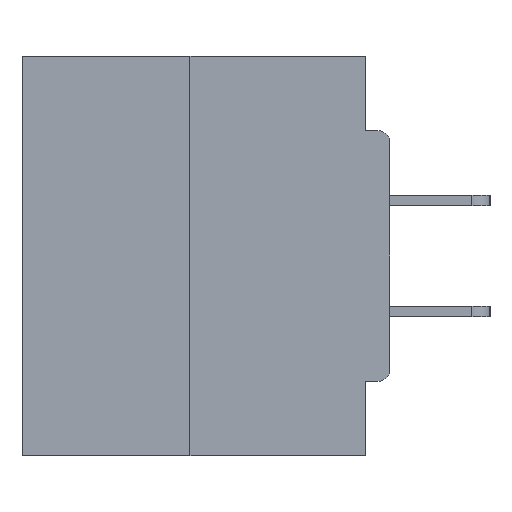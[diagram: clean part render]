
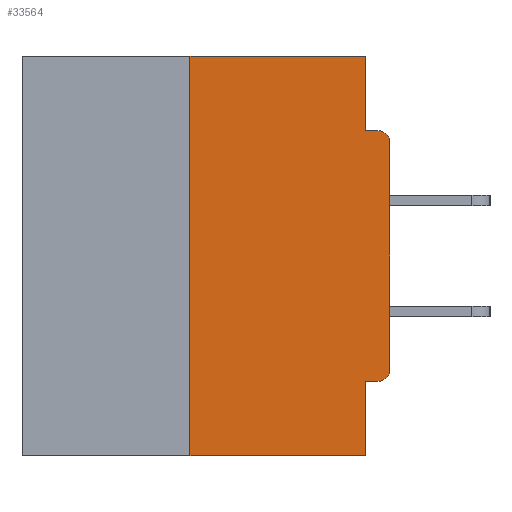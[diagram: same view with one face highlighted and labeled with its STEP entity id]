
A CAD part, left-side view. The second image highlights one B-rep face of the part: STEP entity #33564.
In plain terms, the highlighted planar face has unit normal (-1, 0, 0).
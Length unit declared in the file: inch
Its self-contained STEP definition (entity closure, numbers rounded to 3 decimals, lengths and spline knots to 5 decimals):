
#70 = CIRCLE ( 'NONE', #27551, 0.015 ) ;
#1037 = VERTEX_POINT ( 'NONE', #1949 ) ;
#1400 = LINE ( 'NONE', #12373, #30308 ) ;
#1411 = DIRECTION ( 'NONE',  ( 0., 0., -1. ) ) ;
#1765 = CARTESIAN_POINT ( 'NONE',  ( 0., 0.25, 0. ) ) ;
#1949 = CARTESIAN_POINT ( 'NONE',  ( 0., 0.031, -0.5 ) ) ;
#1954 = CARTESIAN_POINT ( 'NONE',  ( 0., 0.46, 0. ) ) ;
#2030 = EDGE_CURVE ( 'NONE', #9656, #1037, #1400, .T. ) ;
#2289 = ORIENTED_EDGE ( 'NONE', *, *, #35875, .F. ) ;
#2880 = CARTESIAN_POINT ( 'NONE',  ( 0., 0.25, -0.5 ) ) ;
#2998 = VERTEX_POINT ( 'NONE', #32432 ) ;
#3151 = LINE ( 'NONE', #27882, #17383 ) ;
#3451 = CARTESIAN_POINT ( 'NONE',  ( 0., 0.46, 0. ) ) ;
#4517 = DIRECTION ( 'NONE',  ( 1., 0., 0. ) ) ;
#4661 = CARTESIAN_POINT ( 'NONE',  ( 0., 0., -0.4065 ) ) ;
#5572 = ORIENTED_EDGE ( 'NONE', *, *, #20183, .F. ) ;
#7236 = ORIENTED_EDGE ( 'NONE', *, *, #28558, .T. ) ;
#7352 = AXIS2_PLACEMENT_3D ( 'NONE', #29570, #26104, #34522 ) ;
#9108 = DIRECTION ( 'NONE',  ( 0., 0., 1. ) ) ;
#9646 = PLANE ( 'NONE',  #12775 ) ;
#9656 = VERTEX_POINT ( 'NONE', #2880 ) ;
#10022 = VECTOR ( 'NONE', #9108, 39.37008 ) ;
#10520 = LINE ( 'NONE', #4661, #33138 ) ;
#10709 = EDGE_CURVE ( 'NONE', #30648, #2998, #70, .T. ) ;
#10885 = EDGE_CURVE ( 'NONE', #9656, #11603, #18848, .T. ) ;
#11100 = CARTESIAN_POINT ( 'NONE',  ( 0., 0.031, 0. ) ) ;
#11118 = CARTESIAN_POINT ( 'NONE',  ( 0., 0., -0.3915 ) ) ;
#11220 = EDGE_LOOP ( 'NONE', ( #2289, #21263, #24983, #5572, #11323, #7236, #27194, #15880, #24180, #26941 ) ) ;
#11323 = ORIENTED_EDGE ( 'NONE', *, *, #15122, .F. ) ;
#11603 = VERTEX_POINT ( 'NONE', #1765 ) ;
#12114 = CARTESIAN_POINT ( 'NONE',  ( 0., 0.031, -0.4065 ) ) ;
#12373 = CARTESIAN_POINT ( 'NONE',  ( 0., 0.46, -0.5 ) ) ;
#12559 = DIRECTION ( 'NONE',  ( 0., -1., 0. ) ) ;
#12775 = AXIS2_PLACEMENT_3D ( 'NONE', #1954, #4517, #1411 ) ;
#12781 = LINE ( 'NONE', #32939, #34149 ) ;
#14310 = CARTESIAN_POINT ( 'NONE',  ( 0., 0., -0.1085 ) ) ;
#15122 = EDGE_CURVE ( 'NONE', #18452, #19580, #10520, .T. ) ;
#15360 = CARTESIAN_POINT ( 'NONE',  ( 0., 0.015, -0.1085 ) ) ;
#15540 = CIRCLE ( 'NONE', #7352, 0.015 ) ;
#15880 = ORIENTED_EDGE ( 'NONE', *, *, #10709, .T. ) ;
#16033 = CARTESIAN_POINT ( 'NONE',  ( 0., 0.031, -0.0935 ) ) ;
#16152 = EDGE_CURVE ( 'NONE', #31813, #2998, #3151, .T. ) ;
#16269 = EDGE_CURVE ( 'NONE', #17108, #30648, #31341, .T. ) ;
#16673 = VECTOR ( 'NONE', #30691, 39.37008 ) ;
#17108 = VERTEX_POINT ( 'NONE', #11118 ) ;
#17383 = VECTOR ( 'NONE', #30617, 39.37008 ) ;
#17962 = DIRECTION ( 'NONE',  ( 0., 0., 1. ) ) ;
#18189 = CARTESIAN_POINT ( 'NONE',  ( 0., 0.031, 0. ) ) ;
#18452 = VERTEX_POINT ( 'NONE', #28860 ) ;
#18848 = LINE ( 'NONE', #30004, #10022 ) ;
#19001 = LINE ( 'NONE', #11100, #16673 ) ;
#19060 = VERTEX_POINT ( 'NONE', #18189 ) ;
#19580 = VERTEX_POINT ( 'NONE', #12114 ) ;
#20183 = EDGE_CURVE ( 'NONE', #19580, #1037, #12781, .T. ) ;
#21263 = ORIENTED_EDGE ( 'NONE', *, *, #10885, .F. ) ;
#21328 = DIRECTION ( 'NONE',  ( 0., 1., 0. ) ) ;
#23045 = LINE ( 'NONE', #3451, #28576 ) ;
#24147 = DIRECTION ( 'NONE',  ( 0., 0., -1. ) ) ;
#24180 = ORIENTED_EDGE ( 'NONE', *, *, #16152, .F. ) ;
#24983 = ORIENTED_EDGE ( 'NONE', *, *, #2030, .T. ) ;
#26104 = DIRECTION ( 'NONE',  ( -1., 0., 0. ) ) ;
#26484 = FACE_OUTER_BOUND ( 'NONE', #11220, .T. ) ;
#26570 = CARTESIAN_POINT ( 'NONE',  ( 0., 0., 0. ) ) ;
#26941 = ORIENTED_EDGE ( 'NONE', *, *, #28267, .F. ) ;
#27194 = ORIENTED_EDGE ( 'NONE', *, *, #16269, .T. ) ;
#27551 = AXIS2_PLACEMENT_3D ( 'NONE', #15360, #34952, #35869 ) ;
#27882 = CARTESIAN_POINT ( 'NONE',  ( 0., 0., -0.0935 ) ) ;
#28267 = EDGE_CURVE ( 'NONE', #19060, #31813, #19001, .T. ) ;
#28558 = EDGE_CURVE ( 'NONE', #18452, #17108, #15540, .T. ) ;
#28576 = VECTOR ( 'NONE', #33686, 39.37008 ) ;
#28860 = CARTESIAN_POINT ( 'NONE',  ( 0., 0.015, -0.4065 ) ) ;
#29570 = CARTESIAN_POINT ( 'NONE',  ( 0., 0.015, -0.3915 ) ) ;
#30004 = CARTESIAN_POINT ( 'NONE',  ( 0., 0.25, 0. ) ) ;
#30308 = VECTOR ( 'NONE', #12559, 39.37008 ) ;
#30617 = DIRECTION ( 'NONE',  ( 0., -1., 0. ) ) ;
#30648 = VERTEX_POINT ( 'NONE', #14310 ) ;
#30691 = DIRECTION ( 'NONE',  ( 0., 0., -1. ) ) ;
#31341 = LINE ( 'NONE', #26570, #34926 ) ;
#31813 = VERTEX_POINT ( 'NONE', #16033 ) ;
#32432 = CARTESIAN_POINT ( 'NONE',  ( 0., 0.015, -0.0935 ) ) ;
#32939 = CARTESIAN_POINT ( 'NONE',  ( 0., 0.031, -0.5 ) ) ;
#33138 = VECTOR ( 'NONE', #21328, 39.37008 ) ;
#33564 = ADVANCED_FACE ( 'NONE', ( #26484 ), #9646, .F. ) ;
#33686 = DIRECTION ( 'NONE',  ( 0., -1., 0. ) ) ;
#34149 = VECTOR ( 'NONE', #24147, 39.37008 ) ;
#34522 = DIRECTION ( 'NONE',  ( 0., 0., -1. ) ) ;
#34926 = VECTOR ( 'NONE', #17962, 39.37008 ) ;
#34952 = DIRECTION ( 'NONE',  ( -1., 0., 0. ) ) ;
#35869 = DIRECTION ( 'NONE',  ( 0., 0., -1. ) ) ;
#35875 = EDGE_CURVE ( 'NONE', #11603, #19060, #23045, .T. ) ;
